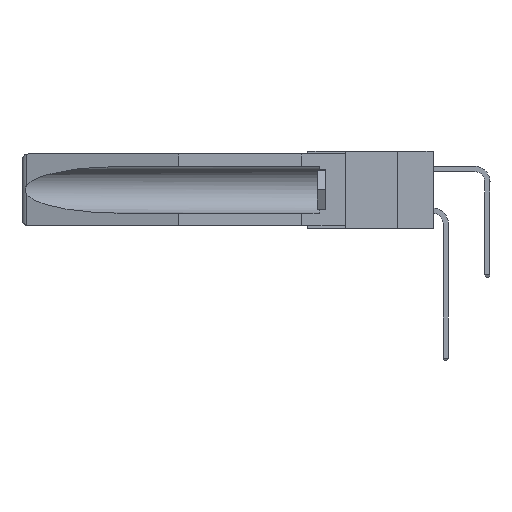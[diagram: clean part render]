
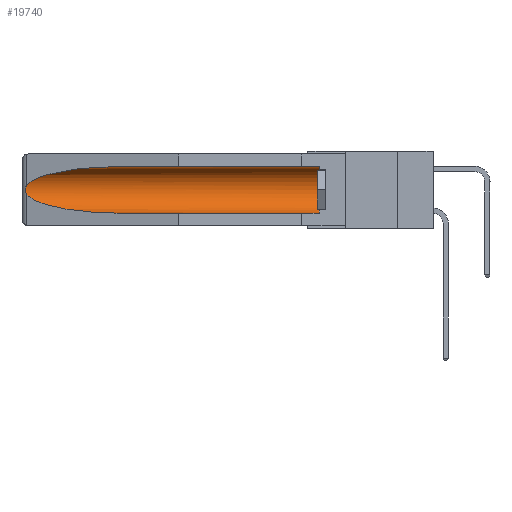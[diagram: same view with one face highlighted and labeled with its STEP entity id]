
A CAD part, left-side view. The second image highlights one B-rep face of the part: STEP entity #19740.
In plain terms, the highlighted cylindrical face has radius 2.857 mm (diameter 5.715 mm), a partial arc.
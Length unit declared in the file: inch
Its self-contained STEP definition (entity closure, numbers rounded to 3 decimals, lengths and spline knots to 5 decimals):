
#1086 = CARTESIAN_POINT ( 'NONE',  ( 0.21114, 1.30732, -0.059 ) ) ;
#1481 = CARTESIAN_POINT ( 'NONE',  ( 0.155, 0.126, -0.284 ) ) ;
#1605 = CIRCLE ( 'NONE', #16677, 0.1125 ) ;
#2570 = ORIENTED_EDGE ( 'NONE', *, *, #13712, .T. ) ;
#2836 = CARTESIAN_POINT ( 'NONE',  ( 0.21114, 1.30732, -0.284 ) ) ;
#2984 = CARTESIAN_POINT ( 'NONE',  ( 0.26655, 1.53094, -0.18657 ) ) ;
#3294 = AXIS2_PLACEMENT_3D ( 'NONE', #6060, #3806, #15214 ) ;
#3761 =( BOUNDED_CURVE ( )  B_SPLINE_CURVE ( 3, ( #25897, #14237, #2836, #18651 ),
 .UNSPECIFIED., .F., .F. ) 
 B_SPLINE_CURVE_WITH_KNOTS ( ( 4, 4 ),
 ( 0.1948, 1.5708 ),
 .UNSPECIFIED. ) 
 CURVE ( )  GEOMETRIC_REPRESENTATION_ITEM ( )  RATIONAL_B_SPLINE_CURVE ( ( 1., 0.848, 0.848, 1. ) ) 
 REPRESENTATION_ITEM ( '' )  );
#3806 = DIRECTION ( 'NONE',  ( 0., 1., 0. ) ) ;
#5849 = CARTESIAN_POINT ( 'NONE',  ( 0.155, 1.07973, -0.284 ) ) ;
#5926 =( BOUNDED_CURVE ( )  B_SPLINE_CURVE ( 3, ( #23675, #1086, #23962, #16886 ),
 .UNSPECIFIED., .F., .F. ) 
 B_SPLINE_CURVE_WITH_KNOTS ( ( 4, 4 ),
 ( 4.71239, 6.08839 ),
 .UNSPECIFIED. ) 
 CURVE ( )  GEOMETRIC_REPRESENTATION_ITEM ( )  RATIONAL_B_SPLINE_CURVE ( ( 1., 0.848, 0.848, 1. ) ) 
 REPRESENTATION_ITEM ( '' )  );
#5981 = ORIENTED_EDGE ( 'NONE', *, *, #8716, .F. ) ;
#6060 = CARTESIAN_POINT ( 'NONE',  ( 0.155, -0.30754, -0.1715 ) ) ;
#7093 = CARTESIAN_POINT ( 'NONE',  ( 0.2673, 1.5327, -0.16383 ) ) ;
#7196 = CARTESIAN_POINT ( 'NONE',  ( 0.26597, 1.5296, -0.19026 ) ) ;
#8716 = EDGE_CURVE ( 'NONE', #14056, #11003, #15813, .T. ) ;
#8995 = CARTESIAN_POINT ( 'NONE',  ( 0.26654, 1.53092, -0.15636 ) ) ;
#9817 = EDGE_CURVE ( 'NONE', #14056, #13142, #1605, .T. ) ;
#10126 = VECTOR ( 'NONE', #15332, 39.37008 ) ;
#11003 = VERTEX_POINT ( 'NONE', #5849 ) ;
#11209 = DIRECTION ( 'NONE',  ( 0., 1., 0. ) ) ;
#11396 = FACE_OUTER_BOUND ( 'NONE', #14649, .T. ) ;
#11568 = LINE ( 'NONE', #22567, #22880 ) ;
#11595 = CARTESIAN_POINT ( 'NONE',  ( 0.2673, 1.53269, -0.17917 ) ) ;
#13142 = VERTEX_POINT ( 'NONE', #24097 ) ;
#13394 = DIRECTION ( 'NONE',  ( 0., 0., 1. ) ) ;
#13712 = EDGE_CURVE ( 'NONE', #21049, #11003, #3761, .T. ) ;
#13793 = VERTEX_POINT ( 'NONE', #18348 ) ;
#14056 = VERTEX_POINT ( 'NONE', #1481 ) ;
#14237 = CARTESIAN_POINT ( 'NONE',  ( 0.25451, 1.48313, -0.24835 ) ) ;
#14649 = EDGE_LOOP ( 'NONE', ( #22695, #25541, #2570, #5981, #23640, #21129 ) ) ;
#14697 = B_SPLINE_CURVE_WITH_KNOTS ( 'NONE', 3,
 ( #25119, #20671, #8995, #7093, #20394, #22654, #11595, #2984, #7196, #25415 ),
 .UNSPECIFIED., .F., .F.,
 ( 4, 2, 2, 2, 4 ),
 ( 0., 0.00029, 0.00058, 0.00087, 0.00117 ),
 .UNSPECIFIED. ) ;
#15214 = DIRECTION ( 'NONE',  ( 0., 0., 1. ) ) ;
#15275 = DIRECTION ( 'NONE',  ( 0., -1., 0. ) ) ;
#15332 = DIRECTION ( 'NONE',  ( 0., 1., 0. ) ) ;
#15643 = CYLINDRICAL_SURFACE ( 'NONE', #3294, 0.1125 ) ;
#15813 = LINE ( 'NONE', #21840, #10126 ) ;
#16677 = AXIS2_PLACEMENT_3D ( 'NONE', #22248, #15275, #13394 ) ;
#16886 = CARTESIAN_POINT ( 'NONE',  ( 0.26537, 1.52718, -0.14972 ) ) ;
#18348 = CARTESIAN_POINT ( 'NONE',  ( 0.26537, 1.52718, -0.14972 ) ) ;
#18651 = CARTESIAN_POINT ( 'NONE',  ( 0.155, 1.07973, -0.284 ) ) ;
#19218 = CARTESIAN_POINT ( 'NONE',  ( 0.155, 1.07973, -0.059 ) ) ;
#19623 = EDGE_CURVE ( 'NONE', #19772, #13793, #5926, .T. ) ;
#19740 = ADVANCED_FACE ( 'NONE', ( #11396 ), #15643, .F. ) ;
#19772 = VERTEX_POINT ( 'NONE', #19218 ) ;
#20394 = CARTESIAN_POINT ( 'NONE',  ( 0.2675, 1.53308, -0.16763 ) ) ;
#20671 = CARTESIAN_POINT ( 'NONE',  ( 0.26597, 1.52961, -0.15275 ) ) ;
#21049 = VERTEX_POINT ( 'NONE', #21561 ) ;
#21129 = ORIENTED_EDGE ( 'NONE', *, *, #24840, .T. ) ;
#21561 = CARTESIAN_POINT ( 'NONE',  ( 0.26537, 1.52718, -0.19328 ) ) ;
#21840 = CARTESIAN_POINT ( 'NONE',  ( 0.155, -0.30754, -0.284 ) ) ;
#22248 = CARTESIAN_POINT ( 'NONE',  ( 0.155, 0.126, -0.1715 ) ) ;
#22567 = CARTESIAN_POINT ( 'NONE',  ( 0.155, -0.30754, -0.059 ) ) ;
#22654 = CARTESIAN_POINT ( 'NONE',  ( 0.2675, 1.53308, -0.17534 ) ) ;
#22695 = ORIENTED_EDGE ( 'NONE', *, *, #19623, .T. ) ;
#22880 = VECTOR ( 'NONE', #11209, 39.37008 ) ;
#23640 = ORIENTED_EDGE ( 'NONE', *, *, #9817, .T. ) ;
#23675 = CARTESIAN_POINT ( 'NONE',  ( 0.155, 1.07973, -0.059 ) ) ;
#23962 = CARTESIAN_POINT ( 'NONE',  ( 0.25451, 1.48313, -0.09465 ) ) ;
#24097 = CARTESIAN_POINT ( 'NONE',  ( 0.155, 0.126, -0.059 ) ) ;
#24840 = EDGE_CURVE ( 'NONE', #13142, #19772, #11568, .T. ) ;
#25119 = CARTESIAN_POINT ( 'NONE',  ( 0.26537, 1.52718, -0.14972 ) ) ;
#25415 = CARTESIAN_POINT ( 'NONE',  ( 0.26537, 1.52718, -0.19328 ) ) ;
#25541 = ORIENTED_EDGE ( 'NONE', *, *, #28091, .T. ) ;
#25897 = CARTESIAN_POINT ( 'NONE',  ( 0.26537, 1.52718, -0.19328 ) ) ;
#28091 = EDGE_CURVE ( 'NONE', #13793, #21049, #14697, .T. ) ;
